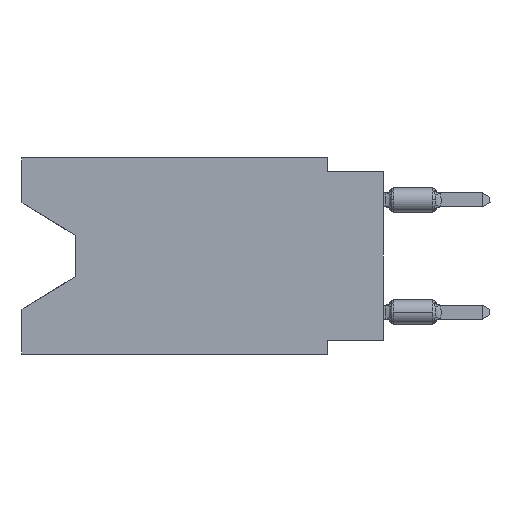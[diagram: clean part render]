
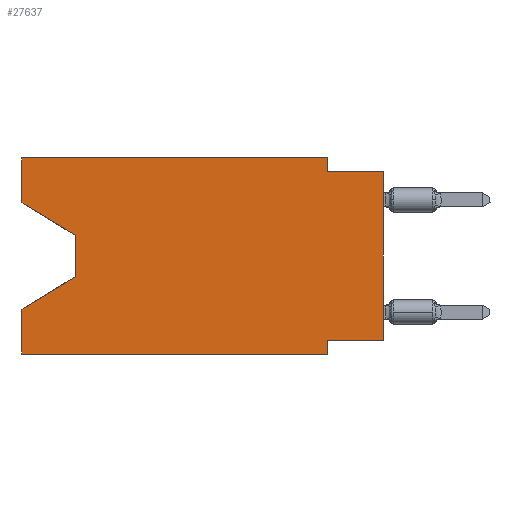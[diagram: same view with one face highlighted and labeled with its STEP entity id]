
A CAD part, left-side view. The second image highlights one B-rep face of the part: STEP entity #27637.
In plain terms, the highlighted planar face has unit normal (-1, 0, 0).
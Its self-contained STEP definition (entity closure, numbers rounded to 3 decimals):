
#102 = CARTESIAN_POINT ( 'NONE',  ( 0., 2.54, -8.255 ) ) ;
#178 = VECTOR ( 'NONE', #49272, 1000. ) ;
#950 = LINE ( 'NONE', #19191, #15618 ) ;
#1517 = EDGE_CURVE ( 'NONE', #34434, #13537, #57935, .T. ) ;
#1673 = LINE ( 'NONE', #14364, #4038 ) ;
#1860 = DIRECTION ( 'NONE',  ( 0., -1., 0. ) ) ;
#2478 = VERTEX_POINT ( 'NONE', #30594 ) ;
#2874 = FACE_OUTER_BOUND ( 'NONE', #3926, .T. ) ;
#3345 = EDGE_CURVE ( 'NONE', #49359, #48431, #1673, .T. ) ;
#3926 = EDGE_LOOP ( 'NONE', ( #42984, #45668, #7748, #25630, #10591, #28460, #43343, #6407, #34861, #29661, #16802, #50319 ) ) ;
#4038 = VECTOR ( 'NONE', #15577, 1000. ) ;
#5063 = VECTOR ( 'NONE', #49258, 1000. ) ;
#6407 = ORIENTED_EDGE ( 'NONE', *, *, #38986, .T. ) ;
#7276 = LINE ( 'NONE', #16262, #178 ) ;
#7435 = EDGE_CURVE ( 'NONE', #54724, #2478, #55040, .T. ) ;
#7748 = ORIENTED_EDGE ( 'NONE', *, *, #3345, .T. ) ;
#8330 = VECTOR ( 'NONE', #57466, 1000. ) ;
#9342 = CARTESIAN_POINT ( 'NONE',  ( 0., 2.54, -8.89 ) ) ;
#9539 = AXIS2_PLACEMENT_3D ( 'NONE', #30997, #26968, #59385 ) ;
#9936 = EDGE_CURVE ( 'NONE', #58309, #19784, #39023, .T. ) ;
#10006 = CARTESIAN_POINT ( 'NONE',  ( 0., 0., -8.255 ) ) ;
#10487 = CARTESIAN_POINT ( 'NONE',  ( 0., 16.383, -8.89 ) ) ;
#10591 = ORIENTED_EDGE ( 'NONE', *, *, #15788, .T. ) ;
#11330 = VERTEX_POINT ( 'NONE', #10006 ) ;
#12253 = CARTESIAN_POINT ( 'NONE',  ( 0., 0., -8.255 ) ) ;
#12789 = LINE ( 'NONE', #41207, #15025 ) ;
#13363 = DIRECTION ( 'NONE',  ( 0., 0., -1. ) ) ;
#13537 = VERTEX_POINT ( 'NONE', #36877 ) ;
#13569 = EDGE_CURVE ( 'NONE', #13537, #42892, #12789, .T. ) ;
#14364 = CARTESIAN_POINT ( 'NONE',  ( 0., 13.97, -5.385 ) ) ;
#14655 = DIRECTION ( 'NONE',  ( 0., -0.855, -0.519 ) ) ;
#14855 = CARTESIAN_POINT ( 'NONE',  ( 0., 16.383, -8.89 ) ) ;
#15025 = VECTOR ( 'NONE', #45537, 1000. ) ;
#15577 = DIRECTION ( 'NONE',  ( 0., 0.855, -0.519 ) ) ;
#15618 = VECTOR ( 'NONE', #28146, 1000. ) ;
#15788 = EDGE_CURVE ( 'NONE', #59200, #2478, #19495, .T. ) ;
#15940 = CARTESIAN_POINT ( 'NONE',  ( 0., 2.54, 0. ) ) ;
#16262 = CARTESIAN_POINT ( 'NONE',  ( 0., 13.97, -3.505 ) ) ;
#16500 = PLANE ( 'NONE',  #9539 ) ;
#16594 = LINE ( 'NONE', #12253, #18297 ) ;
#16802 = ORIENTED_EDGE ( 'NONE', *, *, #51396, .F. ) ;
#16891 = LINE ( 'NONE', #25545, #34633 ) ;
#17492 = DIRECTION ( 'NONE',  ( 0., 1., 0. ) ) ;
#18297 = VECTOR ( 'NONE', #17492, 1000. ) ;
#19191 = CARTESIAN_POINT ( 'NONE',  ( 0., 16.383, 0. ) ) ;
#19495 = LINE ( 'NONE', #14855, #31923 ) ;
#19784 = VERTEX_POINT ( 'NONE', #37952 ) ;
#21085 = EDGE_CURVE ( 'NONE', #59200, #48431, #34009, .T. ) ;
#25545 = CARTESIAN_POINT ( 'NONE',  ( 0., 16.383, 0. ) ) ;
#25630 = ORIENTED_EDGE ( 'NONE', *, *, #21085, .F. ) ;
#25927 = CARTESIAN_POINT ( 'NONE',  ( 0., 0., 0. ) ) ;
#26968 = DIRECTION ( 'NONE',  ( 1., 0., 0. ) ) ;
#27637 = ADVANCED_FACE ( 'NONE', ( #2874 ), #16500, .F. ) ;
#28146 = DIRECTION ( 'NONE',  ( 0., 0., 1. ) ) ;
#28460 = ORIENTED_EDGE ( 'NONE', *, *, #7435, .F. ) ;
#29661 = ORIENTED_EDGE ( 'NONE', *, *, #1517, .F. ) ;
#29953 = DIRECTION ( 'NONE',  ( 0., 0., 1. ) ) ;
#30594 = CARTESIAN_POINT ( 'NONE',  ( 0., 2.54, -8.89 ) ) ;
#30997 = CARTESIAN_POINT ( 'NONE',  ( 0., 16.383, 0. ) ) ;
#31213 = VECTOR ( 'NONE', #29953, 1000. ) ;
#31923 = VECTOR ( 'NONE', #1860, 1000. ) ;
#34009 = LINE ( 'NONE', #52834, #8330 ) ;
#34434 = VERTEX_POINT ( 'NONE', #53593 ) ;
#34633 = VECTOR ( 'NONE', #44379, 1000. ) ;
#34861 = ORIENTED_EDGE ( 'NONE', *, *, #13569, .F. ) ;
#35473 = CARTESIAN_POINT ( 'NONE',  ( 0., 16.383, -6.852 ) ) ;
#36877 = CARTESIAN_POINT ( 'NONE',  ( 0., 2.54, -0.635 ) ) ;
#37172 = VECTOR ( 'NONE', #14655, 1000. ) ;
#37952 = CARTESIAN_POINT ( 'NONE',  ( 0., 13.97, -3.505 ) ) ;
#38986 = EDGE_CURVE ( 'NONE', #11330, #42892, #43543, .T. ) ;
#39023 = LINE ( 'NONE', #57859, #37172 ) ;
#39482 = EDGE_CURVE ( 'NONE', #11330, #54724, #16594, .T. ) ;
#40518 = CARTESIAN_POINT ( 'NONE',  ( 0., 16.383, 0. ) ) ;
#41092 = CARTESIAN_POINT ( 'NONE',  ( 0., 13.97, -5.385 ) ) ;
#41207 = CARTESIAN_POINT ( 'NONE',  ( 0., 0., -0.635 ) ) ;
#42782 = EDGE_CURVE ( 'NONE', #58309, #43583, #950, .T. ) ;
#42892 = VERTEX_POINT ( 'NONE', #44174 ) ;
#42984 = ORIENTED_EDGE ( 'NONE', *, *, #9936, .T. ) ;
#43343 = ORIENTED_EDGE ( 'NONE', *, *, #39482, .F. ) ;
#43543 = LINE ( 'NONE', #25927, #31213 ) ;
#43583 = VERTEX_POINT ( 'NONE', #40518 ) ;
#43892 = VECTOR ( 'NONE', #13363, 1000. ) ;
#44174 = CARTESIAN_POINT ( 'NONE',  ( 0., 0., -0.635 ) ) ;
#44379 = DIRECTION ( 'NONE',  ( 0., -1., 0. ) ) ;
#45537 = DIRECTION ( 'NONE',  ( 0., -1., 0. ) ) ;
#45668 = ORIENTED_EDGE ( 'NONE', *, *, #58652, .T. ) ;
#48431 = VERTEX_POINT ( 'NONE', #35473 ) ;
#49258 = DIRECTION ( 'NONE',  ( 0., 0., -1. ) ) ;
#49272 = DIRECTION ( 'NONE',  ( 0., 0., -1. ) ) ;
#49359 = VERTEX_POINT ( 'NONE', #41092 ) ;
#50319 = ORIENTED_EDGE ( 'NONE', *, *, #42782, .F. ) ;
#50553 = CARTESIAN_POINT ( 'NONE',  ( 0., 16.383, -2.038 ) ) ;
#51396 = EDGE_CURVE ( 'NONE', #43583, #34434, #16891, .T. ) ;
#52834 = CARTESIAN_POINT ( 'NONE',  ( 0., 16.383, 0. ) ) ;
#53593 = CARTESIAN_POINT ( 'NONE',  ( 0., 2.54, 0. ) ) ;
#54724 = VERTEX_POINT ( 'NONE', #102 ) ;
#55040 = LINE ( 'NONE', #9342, #43892 ) ;
#57466 = DIRECTION ( 'NONE',  ( 0., 0., 1. ) ) ;
#57859 = CARTESIAN_POINT ( 'NONE',  ( 0., 16.383, -2.038 ) ) ;
#57935 = LINE ( 'NONE', #15940, #5063 ) ;
#58309 = VERTEX_POINT ( 'NONE', #50553 ) ;
#58652 = EDGE_CURVE ( 'NONE', #19784, #49359, #7276, .T. ) ;
#59200 = VERTEX_POINT ( 'NONE', #10487 ) ;
#59385 = DIRECTION ( 'NONE',  ( 0., 0., -1. ) ) ;
